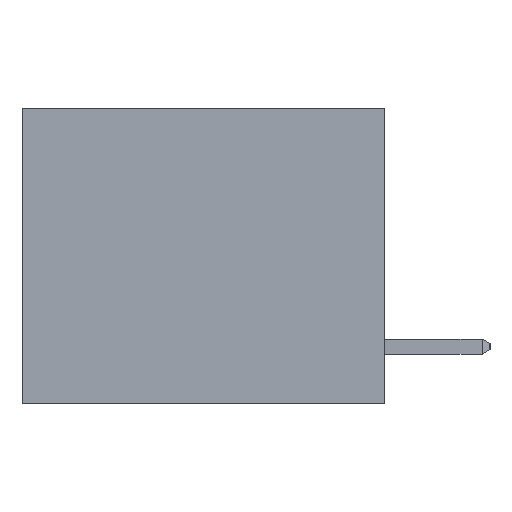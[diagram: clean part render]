
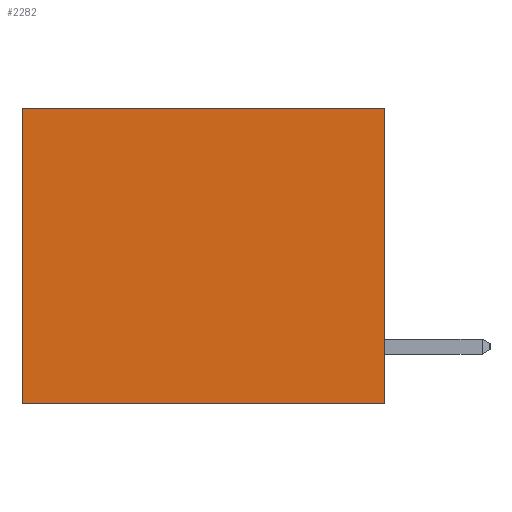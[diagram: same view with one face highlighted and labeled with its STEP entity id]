
A CAD part, left-side view. The second image highlights one B-rep face of the part: STEP entity #2282.
In plain terms, the highlighted planar face has unit normal (-1, 0, 0).
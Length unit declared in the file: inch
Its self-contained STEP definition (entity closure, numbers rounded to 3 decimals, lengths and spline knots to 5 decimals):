
#15 = LINE ( 'NONE', #1983, #23348 ) ;
#1029 = EDGE_CURVE ( 'NONE', #2074, #10842, #3584, .T. ) ;
#1399 = AXIS2_PLACEMENT_3D ( 'NONE', #8507, #6542, #8423 ) ;
#1983 = CARTESIAN_POINT ( 'NONE',  ( 0.3165, 0., 0. ) ) ;
#2074 = VERTEX_POINT ( 'NONE', #17600 ) ;
#2093 = DIRECTION ( 'NONE',  ( 0., 0., -1. ) ) ;
#2282 = ADVANCED_FACE ( 'NONE', ( #8486 ), #12510, .F. ) ;
#2461 = DIRECTION ( 'NONE',  ( 0., 1., 0. ) ) ;
#2660 = DIRECTION ( 'NONE',  ( 0., 1., 0. ) ) ;
#2859 = CARTESIAN_POINT ( 'NONE',  ( 0.3165, 0., -0.49 ) ) ;
#3209 = LINE ( 'NONE', #17557, #17004 ) ;
#3419 = EDGE_CURVE ( 'NONE', #17677, #14698, #3209, .T. ) ;
#3584 = LINE ( 'NONE', #2859, #23844 ) ;
#4915 = DIRECTION ( 'NONE',  ( 0., 0., -1. ) ) ;
#6364 = ORIENTED_EDGE ( 'NONE', *, *, #3419, .T. ) ;
#6500 = CARTESIAN_POINT ( 'NONE',  ( 0.3165, 0.6, 0. ) ) ;
#6542 = DIRECTION ( 'NONE',  ( 1., 0., 0. ) ) ;
#7203 = EDGE_CURVE ( 'NONE', #10842, #14698, #23865, .T. ) ;
#8423 = DIRECTION ( 'NONE',  ( 0., 0., -1. ) ) ;
#8486 = FACE_OUTER_BOUND ( 'NONE', #15527, .T. ) ;
#8507 = CARTESIAN_POINT ( 'NONE',  ( 0.3165, 0., -0.49 ) ) ;
#10842 = VERTEX_POINT ( 'NONE', #14295 ) ;
#11060 = ORIENTED_EDGE ( 'NONE', *, *, #13845, .T. ) ;
#11174 = CARTESIAN_POINT ( 'NONE',  ( 0.3165, 0.6, -0.49 ) ) ;
#12051 = CARTESIAN_POINT ( 'NONE',  ( 0.3165, 0., -0.49 ) ) ;
#12510 = PLANE ( 'NONE',  #1399 ) ;
#13845 = EDGE_CURVE ( 'NONE', #2074, #17677, #15, .T. ) ;
#14295 = CARTESIAN_POINT ( 'NONE',  ( 0.3165, 0., -0.49 ) ) ;
#14698 = VERTEX_POINT ( 'NONE', #11174 ) ;
#15527 = EDGE_LOOP ( 'NONE', ( #6364, #16467, #16565, #11060 ) ) ;
#16467 = ORIENTED_EDGE ( 'NONE', *, *, #7203, .F. ) ;
#16565 = ORIENTED_EDGE ( 'NONE', *, *, #1029, .F. ) ;
#17004 = VECTOR ( 'NONE', #2093, 39.37008 ) ;
#17557 = CARTESIAN_POINT ( 'NONE',  ( 0.3165, 0.6, -0.49 ) ) ;
#17600 = CARTESIAN_POINT ( 'NONE',  ( 0.3165, 0., 0. ) ) ;
#17677 = VERTEX_POINT ( 'NONE', #6500 ) ;
#20810 = VECTOR ( 'NONE', #2461, 39.37008 ) ;
#23348 = VECTOR ( 'NONE', #2660, 39.37008 ) ;
#23844 = VECTOR ( 'NONE', #4915, 39.37008 ) ;
#23865 = LINE ( 'NONE', #12051, #20810 ) ;
